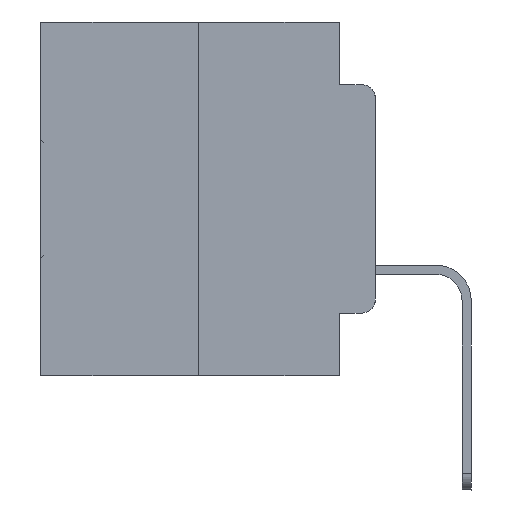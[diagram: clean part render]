
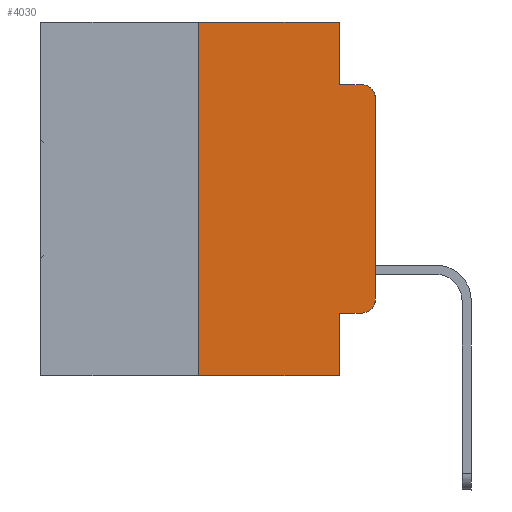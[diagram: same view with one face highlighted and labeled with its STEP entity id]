
A CAD part, left-side view. The second image highlights one B-rep face of the part: STEP entity #4030.
In plain terms, the highlighted planar face has unit normal (-1, 0, 0).
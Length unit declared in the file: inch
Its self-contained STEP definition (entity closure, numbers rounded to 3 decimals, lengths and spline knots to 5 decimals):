
#24 = EDGE_CURVE ( 'NONE', #20418, #26835, #10416, .T. ) ;
#49 = LINE ( 'NONE', #12923, #2738 ) ;
#202 = EDGE_CURVE ( 'NONE', #18904, #1262, #16241, .T. ) ;
#619 = ORIENTED_EDGE ( 'NONE', *, *, #12054, .T. ) ;
#1262 = VERTEX_POINT ( 'NONE', #2482 ) ;
#1426 = ORIENTED_EDGE ( 'NONE', *, *, #29338, .T. ) ;
#1566 = CARTESIAN_POINT ( 'NONE',  ( 0., 0.25, 0. ) ) ;
#1919 = CIRCLE ( 'NONE', #31456, 0.02 ) ;
#2482 = CARTESIAN_POINT ( 'NONE',  ( 0., 0.051, -0.0885 ) ) ;
#2687 = ORIENTED_EDGE ( 'NONE', *, *, #24, .T. ) ;
#2738 = VECTOR ( 'NONE', #20559, 39.37008 ) ;
#3131 = VECTOR ( 'NONE', #26427, 39.37008 ) ;
#3732 = VERTEX_POINT ( 'NONE', #6175 ) ;
#4030 = ADVANCED_FACE ( 'NONE', ( #11451 ), #27576, .F. ) ;
#4047 = CARTESIAN_POINT ( 'NONE',  ( 0., 0.02, -0.1085 ) ) ;
#4168 = VECTOR ( 'NONE', #27087, 39.37008 ) ;
#4248 = CARTESIAN_POINT ( 'NONE',  ( 0., 0.02, -0.4115 ) ) ;
#4518 = EDGE_CURVE ( 'NONE', #11169, #9278, #28498, .T. ) ;
#4546 = CARTESIAN_POINT ( 'NONE',  ( 0., 0., 0. ) ) ;
#4817 = ORIENTED_EDGE ( 'NONE', *, *, #26669, .F. ) ;
#5223 = DIRECTION ( 'NONE',  ( 0., 0., -1. ) ) ;
#6175 = CARTESIAN_POINT ( 'NONE',  ( 0., 0.051, -0.4115 ) ) ;
#6268 = LINE ( 'NONE', #6709, #27674 ) ;
#6465 = EDGE_CURVE ( 'NONE', #3732, #18242, #16385, .T. ) ;
#6709 = CARTESIAN_POINT ( 'NONE',  ( 0., 0.051, -0.4115 ) ) ;
#7558 = CIRCLE ( 'NONE', #16052, 0.02 ) ;
#7693 = DIRECTION ( 'NONE',  ( 0., 0., -1. ) ) ;
#9003 = CARTESIAN_POINT ( 'NONE',  ( 0., 0.051, 0. ) ) ;
#9278 = VERTEX_POINT ( 'NONE', #14869 ) ;
#9644 = EDGE_CURVE ( 'NONE', #26835, #22888, #7558, .T. ) ;
#10416 = LINE ( 'NONE', #4546, #4168 ) ;
#10735 = VERTEX_POINT ( 'NONE', #4248 ) ;
#11169 = VERTEX_POINT ( 'NONE', #25005 ) ;
#11451 = FACE_OUTER_BOUND ( 'NONE', #30745, .T. ) ;
#12047 = VECTOR ( 'NONE', #18635, 39.37008 ) ;
#12054 = EDGE_CURVE ( 'NONE', #10735, #20418, #1919, .T. ) ;
#12458 = CARTESIAN_POINT ( 'NONE',  ( 0., 0.02, -0.0885 ) ) ;
#12691 = CARTESIAN_POINT ( 'NONE',  ( 0., 0.473, 0. ) ) ;
#12923 = CARTESIAN_POINT ( 'NONE',  ( 0., 0.051, -0.0885 ) ) ;
#13084 = CARTESIAN_POINT ( 'NONE',  ( 0., 0.051, 0. ) ) ;
#13926 = CARTESIAN_POINT ( 'NONE',  ( 0., 0., -0.1085 ) ) ;
#14336 = EDGE_CURVE ( 'NONE', #1262, #22888, #49, .T. ) ;
#14785 = CARTESIAN_POINT ( 'NONE',  ( 0., 0.051, 0. ) ) ;
#14869 = CARTESIAN_POINT ( 'NONE',  ( 0., 0.25, 0. ) ) ;
#15039 = ORIENTED_EDGE ( 'NONE', *, *, #14336, .F. ) ;
#15469 = ORIENTED_EDGE ( 'NONE', *, *, #9644, .T. ) ;
#16052 = AXIS2_PLACEMENT_3D ( 'NONE', #4047, #18762, #16364 ) ;
#16241 = LINE ( 'NONE', #14785, #17824 ) ;
#16364 = DIRECTION ( 'NONE',  ( 0., 0., -1. ) ) ;
#16385 = LINE ( 'NONE', #9003, #3131 ) ;
#16476 = DIRECTION ( 'NONE',  ( 0., -1., 0. ) ) ;
#17577 = ORIENTED_EDGE ( 'NONE', *, *, #29826, .T. ) ;
#17824 = VECTOR ( 'NONE', #5223, 39.37008 ) ;
#18242 = VERTEX_POINT ( 'NONE', #25161 ) ;
#18635 = DIRECTION ( 'NONE',  ( 0., -1., 0. ) ) ;
#18762 = DIRECTION ( 'NONE',  ( -1., 0., 0. ) ) ;
#18904 = VERTEX_POINT ( 'NONE', #13084 ) ;
#18985 = DIRECTION ( 'NONE',  ( 0., 0., 1. ) ) ;
#19700 = ORIENTED_EDGE ( 'NONE', *, *, #6465, .F. ) ;
#20181 = CARTESIAN_POINT ( 'NONE',  ( 0., 0., -0.3915 ) ) ;
#20418 = VERTEX_POINT ( 'NONE', #20181 ) ;
#20559 = DIRECTION ( 'NONE',  ( 0., -1., 0. ) ) ;
#21023 = LINE ( 'NONE', #30766, #12047 ) ;
#21128 = ORIENTED_EDGE ( 'NONE', *, *, #4518, .F. ) ;
#21274 = CARTESIAN_POINT ( 'NONE',  ( 0., 0.473, -0.5 ) ) ;
#21744 = CARTESIAN_POINT ( 'NONE',  ( 0., 0.02, -0.3915 ) ) ;
#21749 = AXIS2_PLACEMENT_3D ( 'NONE', #12691, #29950, #7693 ) ;
#22888 = VERTEX_POINT ( 'NONE', #12458 ) ;
#23758 = LINE ( 'NONE', #21274, #31466 ) ;
#23870 = VECTOR ( 'NONE', #18985, 39.37008 ) ;
#24111 = DIRECTION ( 'NONE',  ( 0., -1., 0. ) ) ;
#24239 = DIRECTION ( 'NONE',  ( -1., 0., 0. ) ) ;
#24672 = DIRECTION ( 'NONE',  ( 0., 0., -1. ) ) ;
#25005 = CARTESIAN_POINT ( 'NONE',  ( 0., 0.25, -0.5 ) ) ;
#25161 = CARTESIAN_POINT ( 'NONE',  ( 0., 0.051, -0.5 ) ) ;
#26427 = DIRECTION ( 'NONE',  ( 0., 0., -1. ) ) ;
#26669 = EDGE_CURVE ( 'NONE', #9278, #18904, #21023, .T. ) ;
#26835 = VERTEX_POINT ( 'NONE', #13926 ) ;
#27087 = DIRECTION ( 'NONE',  ( 0., 0., 1. ) ) ;
#27576 = PLANE ( 'NONE',  #21749 ) ;
#27674 = VECTOR ( 'NONE', #24111, 39.37008 ) ;
#28498 = LINE ( 'NONE', #1566, #23870 ) ;
#28668 = ORIENTED_EDGE ( 'NONE', *, *, #202, .F. ) ;
#29338 = EDGE_CURVE ( 'NONE', #3732, #10735, #6268, .T. ) ;
#29826 = EDGE_CURVE ( 'NONE', #11169, #18242, #23758, .T. ) ;
#29950 = DIRECTION ( 'NONE',  ( 1., 0., 0. ) ) ;
#30745 = EDGE_LOOP ( 'NONE', ( #2687, #15469, #15039, #28668, #4817, #21128, #17577, #19700, #1426, #619 ) ) ;
#30766 = CARTESIAN_POINT ( 'NONE',  ( 0., 0.473, 0. ) ) ;
#31456 = AXIS2_PLACEMENT_3D ( 'NONE', #21744, #24239, #24672 ) ;
#31466 = VECTOR ( 'NONE', #16476, 39.37008 ) ;
